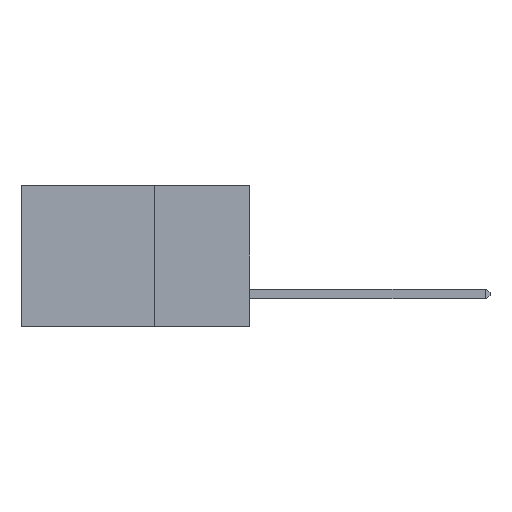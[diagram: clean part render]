
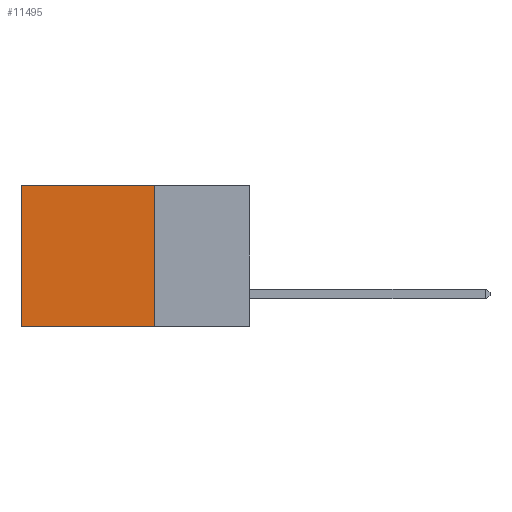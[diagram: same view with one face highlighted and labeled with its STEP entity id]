
A CAD part, left-side view. The second image highlights one B-rep face of the part: STEP entity #11495.
In plain terms, the highlighted planar face has unit normal (-1, 0, 0).
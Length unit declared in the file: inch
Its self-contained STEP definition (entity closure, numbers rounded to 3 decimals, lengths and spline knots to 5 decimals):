
#1807 = LINE ( 'NONE', #10248, #8690 ) ;
#3481 = DIRECTION ( 'NONE',  ( 0., 1., 0. ) ) ;
#3647 = EDGE_CURVE ( 'NONE', #16106, #12456, #6416, .T. ) ;
#4226 = LINE ( 'NONE', #8698, #10956 ) ;
#4432 = CARTESIAN_POINT ( 'NONE',  ( 0.2875, 0.25, 0. ) ) ;
#4600 = EDGE_CURVE ( 'NONE', #9325, #13448, #1807, .T. ) ;
#5249 = PLANE ( 'NONE',  #10824 ) ;
#5332 = CARTESIAN_POINT ( 'NONE',  ( 0.2875, 0.25, 0. ) ) ;
#5595 = DIRECTION ( 'NONE',  ( 0., 1., 0. ) ) ;
#5809 = DIRECTION ( 'NONE',  ( 0., 0., -1. ) ) ;
#6416 = LINE ( 'NONE', #5332, #13844 ) ;
#6417 = ORIENTED_EDGE ( 'NONE', *, *, #3647, .T. ) ;
#7987 = DIRECTION ( 'NONE',  ( 0., 0., -1. ) ) ;
#8690 = VECTOR ( 'NONE', #3481, 39.37008 ) ;
#8698 = CARTESIAN_POINT ( 'NONE',  ( 0.2875, 0.6, 0. ) ) ;
#9268 = LINE ( 'NONE', #4432, #15786 ) ;
#9325 = VERTEX_POINT ( 'NONE', #9739 ) ;
#9739 = CARTESIAN_POINT ( 'NONE',  ( 0.2875, 0.25, -0.37 ) ) ;
#9934 = CARTESIAN_POINT ( 'NONE',  ( 0.2875, 0.6, 0. ) ) ;
#10043 = DIRECTION ( 'NONE',  ( 0., 0., -1. ) ) ;
#10248 = CARTESIAN_POINT ( 'NONE',  ( 0.2875, 0.25, -0.37 ) ) ;
#10726 = EDGE_CURVE ( 'NONE', #12456, #13448, #4226, .T. ) ;
#10824 = AXIS2_PLACEMENT_3D ( 'NONE', #15708, #15822, #7987 ) ;
#10832 = EDGE_LOOP ( 'NONE', ( #15256, #16428, #12163, #6417 ) ) ;
#10956 = VECTOR ( 'NONE', #10043, 39.37008 ) ;
#11495 = ADVANCED_FACE ( 'NONE', ( #14800 ), #5249, .F. ) ;
#12163 = ORIENTED_EDGE ( 'NONE', *, *, #12412, .F. ) ;
#12412 = EDGE_CURVE ( 'NONE', #16106, #9325, #9268, .T. ) ;
#12456 = VERTEX_POINT ( 'NONE', #9934 ) ;
#13108 = CARTESIAN_POINT ( 'NONE',  ( 0.2875, 0.25, 0. ) ) ;
#13448 = VERTEX_POINT ( 'NONE', #16848 ) ;
#13844 = VECTOR ( 'NONE', #5595, 39.37008 ) ;
#14800 = FACE_OUTER_BOUND ( 'NONE', #10832, .T. ) ;
#15256 = ORIENTED_EDGE ( 'NONE', *, *, #10726, .T. ) ;
#15708 = CARTESIAN_POINT ( 'NONE',  ( 0.2875, 0.25, 0. ) ) ;
#15786 = VECTOR ( 'NONE', #5809, 39.37008 ) ;
#15822 = DIRECTION ( 'NONE',  ( 1., 0., 0. ) ) ;
#16106 = VERTEX_POINT ( 'NONE', #13108 ) ;
#16428 = ORIENTED_EDGE ( 'NONE', *, *, #4600, .F. ) ;
#16848 = CARTESIAN_POINT ( 'NONE',  ( 0.2875, 0.6, -0.37 ) ) ;
